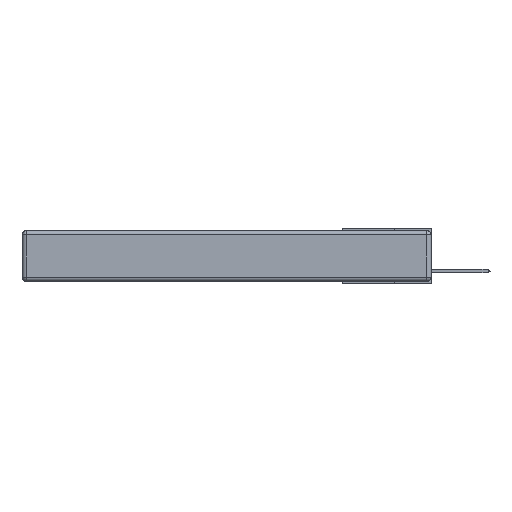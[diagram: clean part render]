
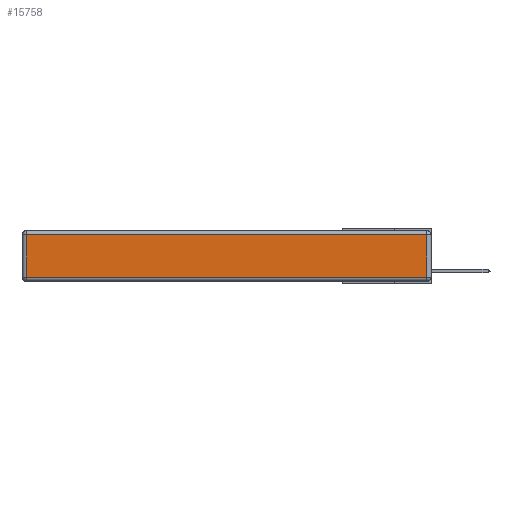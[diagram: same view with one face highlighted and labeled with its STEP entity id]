
A CAD part, left-side view. The second image highlights one B-rep face of the part: STEP entity #15758.
In plain terms, the highlighted planar face has unit normal (-1, 0, 0).
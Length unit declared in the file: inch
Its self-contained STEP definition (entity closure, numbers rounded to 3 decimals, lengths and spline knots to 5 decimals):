
#215 = CARTESIAN_POINT ( 'NONE',  ( 0., 0.03, -0.313 ) ) ;
#615 = DIRECTION ( 'NONE',  ( 0., 0., -1. ) ) ;
#1337 = LINE ( 'NONE', #14582, #16140 ) ;
#1644 = EDGE_CURVE ( 'NONE', #2381, #5883, #3545, .T. ) ;
#2381 = VERTEX_POINT ( 'NONE', #3541 ) ;
#3541 = CARTESIAN_POINT ( 'NONE',  ( 0., 0.03, -0.03 ) ) ;
#3545 = LINE ( 'NONE', #23469, #23151 ) ;
#4847 = DIRECTION ( 'NONE',  ( 0., 0., 1. ) ) ;
#4964 = VERTEX_POINT ( 'NONE', #13391 ) ;
#5563 = ORIENTED_EDGE ( 'NONE', *, *, #17620, .T. ) ;
#5883 = VERTEX_POINT ( 'NONE', #17104 ) ;
#8495 = AXIS2_PLACEMENT_3D ( 'NONE', #17689, #10594, #12102 ) ;
#9735 = CARTESIAN_POINT ( 'NONE',  ( 0., 2.72, -0.343 ) ) ;
#10594 = DIRECTION ( 'NONE',  ( -1., 0., 0. ) ) ;
#10938 = VERTEX_POINT ( 'NONE', #215 ) ;
#11083 = VECTOR ( 'NONE', #4847, 39.37008 ) ;
#12038 = CARTESIAN_POINT ( 'NONE',  ( 0., 0.03, -0.343 ) ) ;
#12102 = DIRECTION ( 'NONE',  ( 0., 0., 1. ) ) ;
#12182 = PLANE ( 'NONE',  #8495 ) ;
#12258 = ORIENTED_EDGE ( 'NONE', *, *, #1644, .T. ) ;
#12799 = EDGE_CURVE ( 'NONE', #10938, #2381, #23270, .T. ) ;
#13391 = CARTESIAN_POINT ( 'NONE',  ( 0., 2.72, -0.313 ) ) ;
#14582 = CARTESIAN_POINT ( 'NONE',  ( 0., 0., -0.313 ) ) ;
#15758 = ADVANCED_FACE ( 'NONE', ( #22586 ), #12182, .T. ) ;
#16140 = VECTOR ( 'NONE', #16402, 39.37008 ) ;
#16402 = DIRECTION ( 'NONE',  ( 0., -1., 0. ) ) ;
#17104 = CARTESIAN_POINT ( 'NONE',  ( 0., 2.72, -0.03 ) ) ;
#17181 = EDGE_CURVE ( 'NONE', #5883, #4964, #18113, .T. ) ;
#17620 = EDGE_CURVE ( 'NONE', #4964, #10938, #1337, .T. ) ;
#17689 = CARTESIAN_POINT ( 'NONE',  ( 0., 0., -0.343 ) ) ;
#17982 = DIRECTION ( 'NONE',  ( 0., 1., 0. ) ) ;
#18113 = LINE ( 'NONE', #9735, #21251 ) ;
#19194 = ORIENTED_EDGE ( 'NONE', *, *, #17181, .T. ) ;
#21005 = EDGE_LOOP ( 'NONE', ( #5563, #23249, #12258, #19194 ) ) ;
#21251 = VECTOR ( 'NONE', #615, 39.37008 ) ;
#22586 = FACE_OUTER_BOUND ( 'NONE', #21005, .T. ) ;
#23151 = VECTOR ( 'NONE', #17982, 39.37008 ) ;
#23249 = ORIENTED_EDGE ( 'NONE', *, *, #12799, .T. ) ;
#23270 = LINE ( 'NONE', #12038, #11083 ) ;
#23469 = CARTESIAN_POINT ( 'NONE',  ( 0., 2.75, -0.03 ) ) ;
